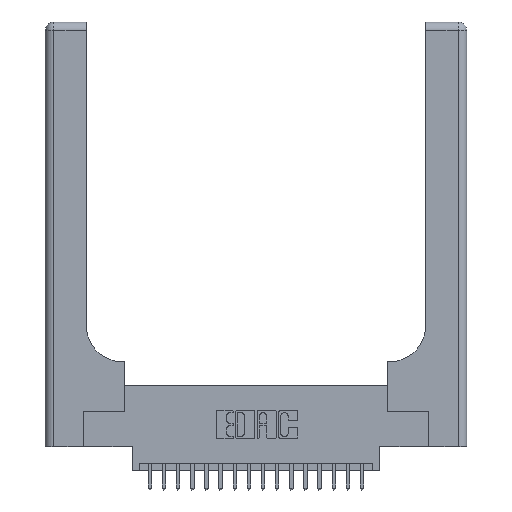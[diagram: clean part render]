
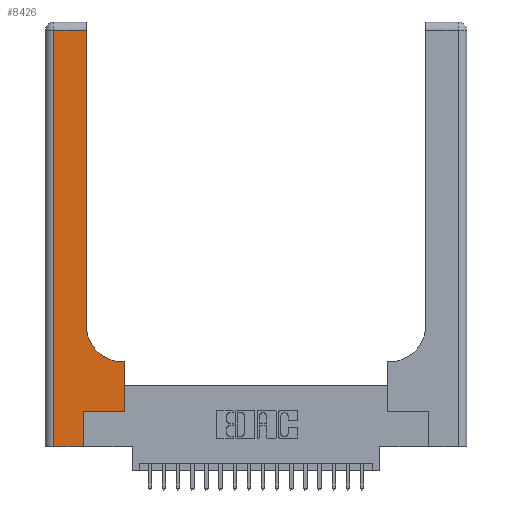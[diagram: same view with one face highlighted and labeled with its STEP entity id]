
A CAD part, top view. The second image highlights one B-rep face of the part: STEP entity #8426.
In plain terms, the highlighted planar face has unit normal (0, 0, 1).
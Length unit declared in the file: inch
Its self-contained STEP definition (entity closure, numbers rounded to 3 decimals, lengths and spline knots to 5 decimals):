
#349 = ORIENTED_EDGE ( 'NONE', *, *, #2376, .T. ) ;
#582 = VERTEX_POINT ( 'NONE', #3898 ) ;
#674 = DIRECTION ( 'NONE',  ( 0., -1., 0. ) ) ;
#1616 = DIRECTION ( 'NONE',  ( 0., 0., -1. ) ) ;
#2104 = ORIENTED_EDGE ( 'NONE', *, *, #18603, .T. ) ;
#2231 = FACE_OUTER_BOUND ( 'NONE', #19364, .T. ) ;
#2358 = VECTOR ( 'NONE', #3713, 39.37008 ) ;
#2376 = EDGE_CURVE ( 'NONE', #17524, #20495, #5999, .T. ) ;
#2511 = VECTOR ( 'NONE', #13271, 39.37008 ) ;
#2988 = VERTEX_POINT ( 'NONE', #6275 ) ;
#3106 = AXIS2_PLACEMENT_3D ( 'NONE', #16052, #6248, #17705 ) ;
#3129 = DIRECTION ( 'NONE',  ( -1., 0., 0. ) ) ;
#3156 = ORIENTED_EDGE ( 'NONE', *, *, #15121, .T. ) ;
#3506 = ORIENTED_EDGE ( 'NONE', *, *, #9446, .T. ) ;
#3713 = DIRECTION ( 'NONE',  ( 0., 1., 0. ) ) ;
#3877 = CARTESIAN_POINT ( 'NONE',  ( 0.2915, 0.85, 0.37 ) ) ;
#3898 = CARTESIAN_POINT ( 'NONE',  ( 0.5585, 0.6, 0.37 ) ) ;
#4575 = PLANE ( 'NONE',  #3106 ) ;
#5069 = LINE ( 'NONE', #18583, #9487 ) ;
#5596 = EDGE_CURVE ( 'NONE', #20495, #17852, #6807, .T. ) ;
#5999 = LINE ( 'NONE', #6303, #8862 ) ;
#6248 = DIRECTION ( 'NONE',  ( 0., 0., -1. ) ) ;
#6275 = CARTESIAN_POINT ( 'NONE',  ( 0.06, 2.94, 0.37 ) ) ;
#6303 = CARTESIAN_POINT ( 'NONE',  ( 0., 0., 0.37 ) ) ;
#6708 = VERTEX_POINT ( 'NONE', #15040 ) ;
#6807 = LINE ( 'NONE', #13490, #2358 ) ;
#7135 = DIRECTION ( 'NONE',  ( 1., 0., 0. ) ) ;
#7160 = ORIENTED_EDGE ( 'NONE', *, *, #21307, .T. ) ;
#7804 = DIRECTION ( 'NONE',  ( 0., 1., 0. ) ) ;
#8426 = ADVANCED_FACE ( 'NONE', ( #2231 ), #4575, .F. ) ;
#8451 = LINE ( 'NONE', #17242, #16093 ) ;
#8862 = VECTOR ( 'NONE', #12810, 39.37008 ) ;
#9446 = EDGE_CURVE ( 'NONE', #2988, #17524, #8451, .T. ) ;
#9487 = VECTOR ( 'NONE', #7135, 39.37008 ) ;
#9728 = ORIENTED_EDGE ( 'NONE', *, *, #13377, .T. ) ;
#10714 = DIRECTION ( 'NONE',  ( 0., 1., 0. ) ) ;
#11310 = ORIENTED_EDGE ( 'NONE', *, *, #5596, .T. ) ;
#11318 = LINE ( 'NONE', #11648, #2511 ) ;
#11499 = LINE ( 'NONE', #14280, #19682 ) ;
#11544 = CARTESIAN_POINT ( 'NONE',  ( 0.5415, 0.85, 0.37 ) ) ;
#11648 = CARTESIAN_POINT ( 'NONE',  ( 0.2915, 0.6, 0.37 ) ) ;
#11881 = CARTESIAN_POINT ( 'NONE',  ( 0.269, 0., 0.37 ) ) ;
#12460 = LINE ( 'NONE', #18864, #20670 ) ;
#12766 = CARTESIAN_POINT ( 'NONE',  ( 0.5585, 0.25, 0.37 ) ) ;
#12810 = DIRECTION ( 'NONE',  ( 1., 0., 0. ) ) ;
#13138 = CARTESIAN_POINT ( 'NONE',  ( 0.06, 0., 0.37 ) ) ;
#13167 = DIRECTION ( 'NONE',  ( 1., 0., 0. ) ) ;
#13271 = DIRECTION ( 'NONE',  ( -1., 0., 0. ) ) ;
#13377 = EDGE_CURVE ( 'NONE', #6708, #2988, #17701, .T. ) ;
#13474 = EDGE_CURVE ( 'NONE', #582, #17707, #11318, .T. ) ;
#13490 = CARTESIAN_POINT ( 'NONE',  ( 0.269, 0., 0.37 ) ) ;
#14280 = CARTESIAN_POINT ( 'NONE',  ( 0.5585, 0.25, 0.37 ) ) ;
#14607 = CIRCLE ( 'NONE', #17128, 0.25 ) ;
#14650 = CARTESIAN_POINT ( 'NONE',  ( 0., 2.94, 0.37 ) ) ;
#14888 = VERTEX_POINT ( 'NONE', #3877 ) ;
#15040 = CARTESIAN_POINT ( 'NONE',  ( 0.2915, 2.94, 0.37 ) ) ;
#15121 = EDGE_CURVE ( 'NONE', #17973, #582, #11499, .T. ) ;
#15430 = CARTESIAN_POINT ( 'NONE',  ( 0.5415, 0.6, 0.37 ) ) ;
#16052 = CARTESIAN_POINT ( 'NONE',  ( 0., 3., 0.37 ) ) ;
#16093 = VECTOR ( 'NONE', #674, 39.37008 ) ;
#17128 = AXIS2_PLACEMENT_3D ( 'NONE', #11544, #1616, #13167 ) ;
#17242 = CARTESIAN_POINT ( 'NONE',  ( 0.06, 3., 0.37 ) ) ;
#17367 = CARTESIAN_POINT ( 'NONE',  ( 0.269, 0.25, 0.37 ) ) ;
#17524 = VERTEX_POINT ( 'NONE', #13138 ) ;
#17701 = LINE ( 'NONE', #14650, #18225 ) ;
#17705 = DIRECTION ( 'NONE',  ( -1., 0., 0. ) ) ;
#17707 = VERTEX_POINT ( 'NONE', #15430 ) ;
#17852 = VERTEX_POINT ( 'NONE', #17367 ) ;
#17973 = VERTEX_POINT ( 'NONE', #12766 ) ;
#18225 = VECTOR ( 'NONE', #3129, 39.37008 ) ;
#18583 = CARTESIAN_POINT ( 'NONE',  ( 0.269, 0.25, 0.37 ) ) ;
#18603 = EDGE_CURVE ( 'NONE', #17707, #14888, #14607, .T. ) ;
#18864 = CARTESIAN_POINT ( 'NONE',  ( 0.2915, 3., 0.37 ) ) ;
#19364 = EDGE_LOOP ( 'NONE', ( #7160, #9728, #3506, #349, #11310, #20538, #3156, #19474, #2104 ) ) ;
#19375 = EDGE_CURVE ( 'NONE', #17852, #17973, #5069, .T. ) ;
#19474 = ORIENTED_EDGE ( 'NONE', *, *, #13474, .T. ) ;
#19682 = VECTOR ( 'NONE', #7804, 39.37008 ) ;
#20495 = VERTEX_POINT ( 'NONE', #11881 ) ;
#20538 = ORIENTED_EDGE ( 'NONE', *, *, #19375, .T. ) ;
#20670 = VECTOR ( 'NONE', #10714, 39.37008 ) ;
#21307 = EDGE_CURVE ( 'NONE', #14888, #6708, #12460, .T. ) ;
